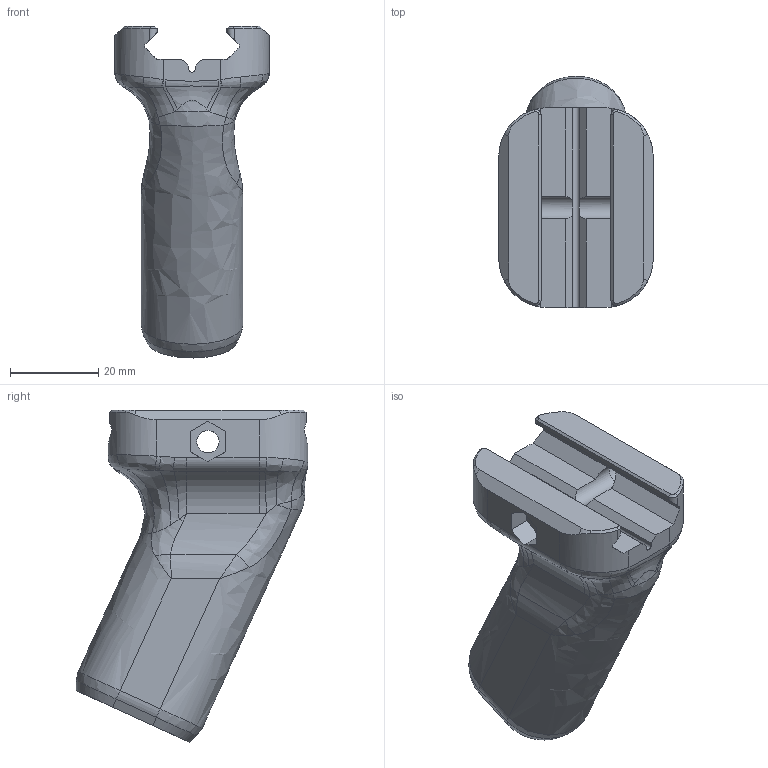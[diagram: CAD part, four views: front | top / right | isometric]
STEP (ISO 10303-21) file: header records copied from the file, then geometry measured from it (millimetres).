
FILE_DESCRIPTION(/* description */ (''),/* implementation_level */ '2;1');
FILE_NAME(/* name */ 'Standard Grip.step',/* time_stamp */ '2021-04-11T01:04:38-04:00',/* author */ (''),/* organization */ (''),/* preprocessor_version */ 'ST-DEVELOPER v18.1',/* originating_system */ 'Autodesk Translation Framework v10.6.0.1341',/* authorisation */ '');
FILE_SCHEMA (('AUTOMOTIVE_DESIGN { 1 0 10303 214 3 1 1 }'));
Length unit declared in the file: millimetre
Products named in the file (1): Standard Grip
Bounding box: 35 x 52.51 x 75.31 mm (x, y, z)
Volume: 32378.3 mm3; surface area: 14346.7 mm2
Topology: 1 solids, 1 shells, 201 faces, 502 edges, 294 vertices
Faces by surface type: bspline 112, plane 50, cylinder 31, cone 8
Full cylindrical faces by diameter (mm): 5.1 x2, 8.75 x1
Entity records: 8637 total; most frequent: CARTESIAN_POINT 4520, ORIENTED_EDGE 988, DIRECTION 615, EDGE_CURVE 494, VERTEX_POINT 294, AXIS2_PLACEMENT_3D 235, B_SPLINE_CURVE_WITH_KNOTS 204, EDGE_LOOP 204
